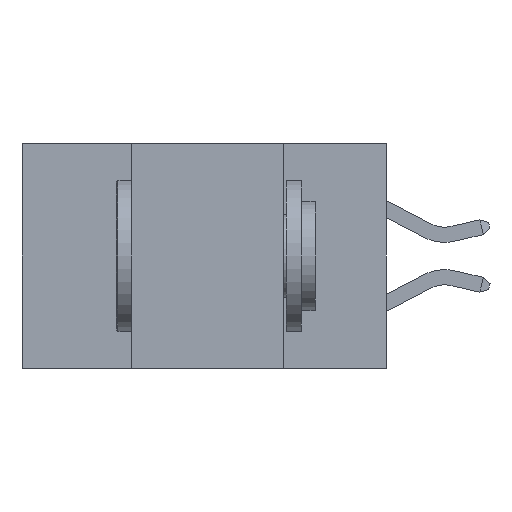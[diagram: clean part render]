
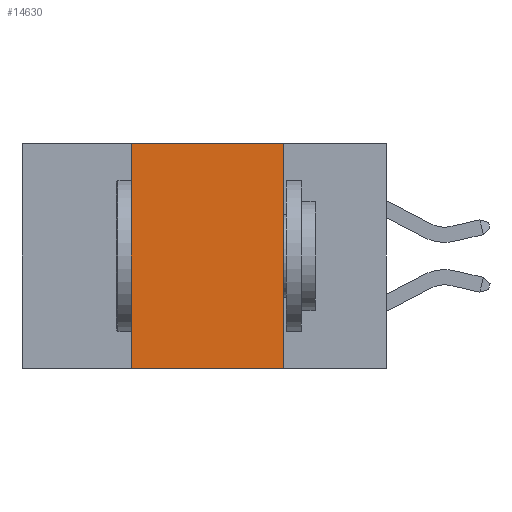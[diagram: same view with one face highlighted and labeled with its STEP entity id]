
A CAD part, left-side view. The second image highlights one B-rep face of the part: STEP entity #14630.
In plain terms, the highlighted planar face has unit normal (-1, 0, 0).
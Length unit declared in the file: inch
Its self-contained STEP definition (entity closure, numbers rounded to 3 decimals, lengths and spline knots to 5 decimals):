
#88 = VECTOR ( 'NONE', #4755, 39.37008 ) ;
#784 = LINE ( 'NONE', #1374, #12654 ) ;
#789 = DIRECTION ( 'NONE',  ( 0., -1., 0. ) ) ;
#897 = CARTESIAN_POINT ( 'NONE',  ( 0., 0.6, 0. ) ) ;
#971 = CARTESIAN_POINT ( 'NONE',  ( 0., 0.42, -0.37 ) ) ;
#997 = DIRECTION ( 'NONE',  ( 0., -1., 0. ) ) ;
#1240 = EDGE_CURVE ( 'NONE', #9075, #9790, #13713, .T. ) ;
#1374 = CARTESIAN_POINT ( 'NONE',  ( 0., 0.6, -0.37 ) ) ;
#1636 = DIRECTION ( 'NONE',  ( 0., 0., -1. ) ) ;
#1656 = DIRECTION ( 'NONE',  ( 1., 0., 0. ) ) ;
#1703 = CARTESIAN_POINT ( 'NONE',  ( 0., 0.6, 0. ) ) ;
#1720 = PLANE ( 'NONE',  #8815 ) ;
#2562 = EDGE_LOOP ( 'NONE', ( #4155, #10536, #12404, #13752 ) ) ;
#3021 = DIRECTION ( 'NONE',  ( 0., 0., 1. ) ) ;
#3316 = VERTEX_POINT ( 'NONE', #13648 ) ;
#3466 = CARTESIAN_POINT ( 'NONE',  ( 0., 0.17, -0.37 ) ) ;
#4155 = ORIENTED_EDGE ( 'NONE', *, *, #10871, .F. ) ;
#4636 = VECTOR ( 'NONE', #3021, 39.37008 ) ;
#4755 = DIRECTION ( 'NONE',  ( 0., 0., -1. ) ) ;
#4907 = CARTESIAN_POINT ( 'NONE',  ( 0., 0.17, -0.37 ) ) ;
#5057 = CARTESIAN_POINT ( 'NONE',  ( 0., 0.42, -0.37 ) ) ;
#6142 = CARTESIAN_POINT ( 'NONE',  ( 0., 0.42, 0. ) ) ;
#6818 = VERTEX_POINT ( 'NONE', #3466 ) ;
#7749 = EDGE_CURVE ( 'NONE', #9075, #6818, #784, .T. ) ;
#8815 = AXIS2_PLACEMENT_3D ( 'NONE', #1703, #1656, #1636 ) ;
#9075 = VERTEX_POINT ( 'NONE', #971 ) ;
#9790 = VERTEX_POINT ( 'NONE', #6142 ) ;
#10536 = ORIENTED_EDGE ( 'NONE', *, *, #13072, .F. ) ;
#10537 = VECTOR ( 'NONE', #789, 39.37008 ) ;
#10871 = EDGE_CURVE ( 'NONE', #3316, #6818, #12681, .T. ) ;
#10884 = LINE ( 'NONE', #897, #10537 ) ;
#11872 = FACE_OUTER_BOUND ( 'NONE', #2562, .T. ) ;
#12404 = ORIENTED_EDGE ( 'NONE', *, *, #1240, .F. ) ;
#12654 = VECTOR ( 'NONE', #997, 39.37008 ) ;
#12681 = LINE ( 'NONE', #4907, #88 ) ;
#13072 = EDGE_CURVE ( 'NONE', #9790, #3316, #10884, .T. ) ;
#13648 = CARTESIAN_POINT ( 'NONE',  ( 0., 0.17, 0. ) ) ;
#13713 = LINE ( 'NONE', #5057, #4636 ) ;
#13752 = ORIENTED_EDGE ( 'NONE', *, *, #7749, .T. ) ;
#14630 = ADVANCED_FACE ( 'NONE', ( #11872 ), #1720, .F. ) ;
